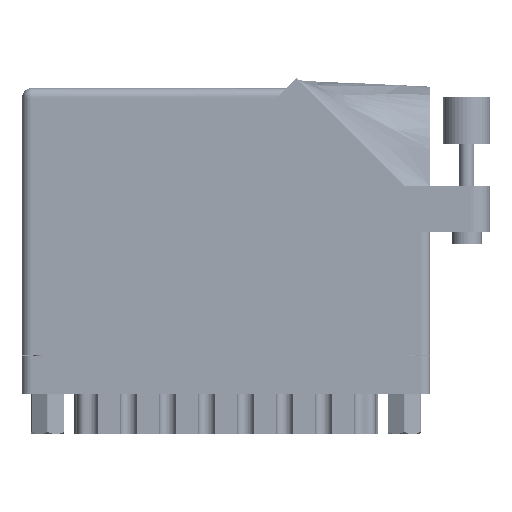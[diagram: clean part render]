
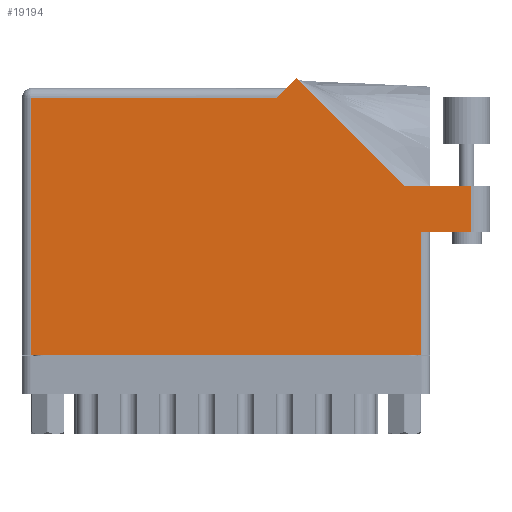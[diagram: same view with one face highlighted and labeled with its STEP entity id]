
A CAD part, front view. The second image highlights one B-rep face of the part: STEP entity #19194.
In plain terms, the highlighted face is planar.
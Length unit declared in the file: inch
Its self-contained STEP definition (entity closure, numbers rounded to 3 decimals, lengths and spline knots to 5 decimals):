
#1396 = LINE ( 'NONE', #24563, #57473 ) ;
#1485 = CARTESIAN_POINT ( 'NONE',  ( 2.993, 1.122, 0. ) ) ;
#2403 = EDGE_CURVE ( 'NONE', #30852, #57801, #6251, .T. ) ;
#2708 = CARTESIAN_POINT ( 'NONE',  ( 0.062, 0., 0. ) ) ;
#3812 = DIRECTION ( 'NONE',  ( 0., 1., 0. ) ) ;
#4975 = EDGE_CURVE ( 'NONE', #5379, #30852, #26713, .T. ) ;
#5379 = VERTEX_POINT ( 'NONE', #26800 ) ;
#5870 = CARTESIAN_POINT ( 'NONE',  ( 1.82871, 1.84571, 0. ) ) ;
#5954 = CARTESIAN_POINT ( 'NONE',  ( 2.993, 0.815, 0. ) ) ;
#6251 = LINE ( 'NONE', #1485, #15559 ) ;
#8669 = CARTESIAN_POINT ( 'NONE',  ( 0., 1.775, 0. ) ) ;
#9202 = VECTOR ( 'NONE', #64489, 39.37008 ) ;
#10348 = EDGE_CURVE ( 'NONE', #23332, #41330, #15396, .T. ) ;
#12179 = VECTOR ( 'NONE', #31865, 39.37008 ) ;
#13330 = VERTEX_POINT ( 'NONE', #83997 ) ;
#14569 = VECTOR ( 'NONE', #56480, 39.37008 ) ;
#15073 = EDGE_CURVE ( 'NONE', #13330, #5379, #63906, .T. ) ;
#15396 = LINE ( 'NONE', #51144, #19592 ) ;
#15559 = VECTOR ( 'NONE', #80799, 39.37008 ) ;
#16641 = ORIENTED_EDGE ( 'NONE', *, *, #15073, .T. ) ;
#18262 = EDGE_CURVE ( 'NONE', #57801, #52871, #85237, .T. ) ;
#18743 = VERTEX_POINT ( 'NONE', #47449 ) ;
#19194 = ADVANCED_FACE ( 'NONE', ( #64271 ), #28687, .F. ) ;
#19592 = VECTOR ( 'NONE', #30524, 39.37008 ) ;
#23070 = DIRECTION ( 'NONE',  ( 1., 0., 0. ) ) ;
#23149 = CARTESIAN_POINT ( 'NONE',  ( 0.062, 1.713, 0. ) ) ;
#23332 = VERTEX_POINT ( 'NONE', #23149 ) ;
#23377 = CARTESIAN_POINT ( 'NONE',  ( 3.118, 1.122, 0. ) ) ;
#23926 = ORIENTED_EDGE ( 'NONE', *, *, #2403, .T. ) ;
#24563 = CARTESIAN_POINT ( 'NONE',  ( 0., 1.713, 0. ) ) ;
#25488 = VECTOR ( 'NONE', #3812, 39.37008 ) ;
#26713 = LINE ( 'NONE', #76670, #12179 ) ;
#26800 = CARTESIAN_POINT ( 'NONE',  ( 2.656, 0.815, 0. ) ) ;
#28687 = PLANE ( 'NONE',  #75205 ) ;
#30524 = DIRECTION ( 'NONE',  ( 0., -1., 0. ) ) ;
#30852 = VERTEX_POINT ( 'NONE', #5954 ) ;
#31865 = DIRECTION ( 'NONE',  ( 1., 0., 0. ) ) ;
#33537 = DIRECTION ( 'NONE',  ( -0.707, -0.707, 0. ) ) ;
#34801 = DIRECTION ( 'NONE',  ( 0., 0., -1. ) ) ;
#35079 = EDGE_CURVE ( 'NONE', #52871, #64472, #40404, .T. ) ;
#39367 = CARTESIAN_POINT ( 'NONE',  ( 1.758, 1.775, 0. ) ) ;
#40404 = LINE ( 'NONE', #77887, #9202 ) ;
#41330 = VERTEX_POINT ( 'NONE', #2708 ) ;
#41891 = LINE ( 'NONE', #39367, #84430 ) ;
#42148 = CARTESIAN_POINT ( 'NONE',  ( 2.993, 1.122, 0. ) ) ;
#43640 = CARTESIAN_POINT ( 'NONE',  ( 2.656, 0.815, 0. ) ) ;
#43926 = VECTOR ( 'NONE', #23070, 39.37008 ) ;
#47149 = EDGE_CURVE ( 'NONE', #41330, #13330, #82349, .T. ) ;
#47449 = CARTESIAN_POINT ( 'NONE',  ( 1.696, 1.713, 0. ) ) ;
#48442 = ORIENTED_EDGE ( 'NONE', *, *, #4975, .T. ) ;
#48892 = CARTESIAN_POINT ( 'NONE',  ( 2.55242, 1.122, 0. ) ) ;
#51144 = CARTESIAN_POINT ( 'NONE',  ( 0.062, 0., 0. ) ) ;
#51273 = DIRECTION ( 'NONE',  ( -1., 0., 0. ) ) ;
#52871 = VERTEX_POINT ( 'NONE', #48892 ) ;
#54711 = ORIENTED_EDGE ( 'NONE', *, *, #18262, .T. ) ;
#56449 = CARTESIAN_POINT ( 'NONE',  ( 0., 0., 0. ) ) ;
#56480 = DIRECTION ( 'NONE',  ( -1., 0., 0. ) ) ;
#57473 = VECTOR ( 'NONE', #51273, 39.37008 ) ;
#57801 = VERTEX_POINT ( 'NONE', #42148 ) ;
#62604 = ORIENTED_EDGE ( 'NONE', *, *, #78012, .T. ) ;
#62747 = ORIENTED_EDGE ( 'NONE', *, *, #67700, .T. ) ;
#62773 = ORIENTED_EDGE ( 'NONE', *, *, #10348, .T. ) ;
#63906 = LINE ( 'NONE', #43640, #25488 ) ;
#64271 = FACE_OUTER_BOUND ( 'NONE', #83630, .T. ) ;
#64472 = VERTEX_POINT ( 'NONE', #5870 ) ;
#64489 = DIRECTION ( 'NONE',  ( -0.707, 0.707, 0. ) ) ;
#67700 = EDGE_CURVE ( 'NONE', #18743, #23332, #1396, .T. ) ;
#74929 = DIRECTION ( 'NONE',  ( -1., 0., 0. ) ) ;
#75205 = AXIS2_PLACEMENT_3D ( 'NONE', #8669, #34801, #74929 ) ;
#76670 = CARTESIAN_POINT ( 'NONE',  ( 2.718, 0.815, 0. ) ) ;
#77887 = CARTESIAN_POINT ( 'NONE',  ( 2.55242, 1.122, 0. ) ) ;
#78012 = EDGE_CURVE ( 'NONE', #64472, #18743, #41891, .T. ) ;
#80799 = DIRECTION ( 'NONE',  ( 0., 1., 0. ) ) ;
#82349 = LINE ( 'NONE', #56449, #43926 ) ;
#83361 = ORIENTED_EDGE ( 'NONE', *, *, #47149, .T. ) ;
#83630 = EDGE_LOOP ( 'NONE', ( #48442, #23926, #54711, #84916, #62604, #62747, #62773, #83361, #16641 ) ) ;
#83997 = CARTESIAN_POINT ( 'NONE',  ( 2.656, 0., 0. ) ) ;
#84430 = VECTOR ( 'NONE', #33537, 39.37008 ) ;
#84916 = ORIENTED_EDGE ( 'NONE', *, *, #35079, .T. ) ;
#85237 = LINE ( 'NONE', #23377, #14569 ) ;
